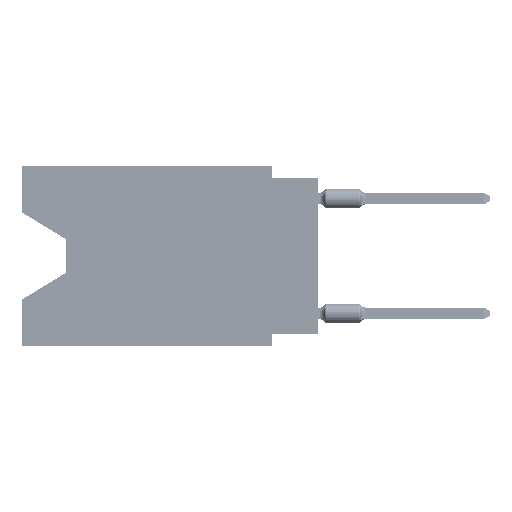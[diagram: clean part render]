
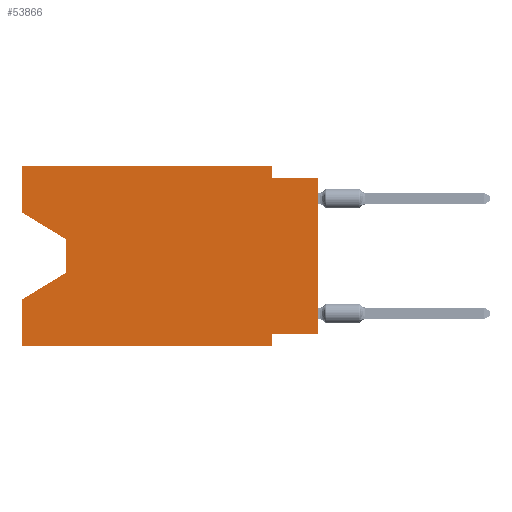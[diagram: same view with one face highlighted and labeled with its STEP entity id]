
A CAD part, left-side view. The second image highlights one B-rep face of the part: STEP entity #53866.
In plain terms, the highlighted planar face has unit normal (-1, 0, 0).
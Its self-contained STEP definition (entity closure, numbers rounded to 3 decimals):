
#454 = ORIENTED_EDGE ( 'NONE', *, *, #25153, .F. ) ;
#1083 = ORIENTED_EDGE ( 'NONE', *, *, #26147, .T. ) ;
#2957 = LINE ( 'NONE', #27052, #9145 ) ;
#4261 = LINE ( 'NONE', #43544, #16232 ) ;
#5022 = LINE ( 'NONE', #71385, #45654 ) ;
#5476 = CARTESIAN_POINT ( 'NONE',  ( 0., 16.383, 0. ) ) ;
#5584 = ORIENTED_EDGE ( 'NONE', *, *, #6152, .T. ) ;
#5935 = CARTESIAN_POINT ( 'NONE',  ( 0., 2.54, 0. ) ) ;
#5943 = DIRECTION ( 'NONE',  ( 0., 0., -1. ) ) ;
#5999 = DIRECTION ( 'NONE',  ( 0., 0., 1. ) ) ;
#6152 = EDGE_CURVE ( 'NONE', #68280, #65793, #2957, .T. ) ;
#6494 = VECTOR ( 'NONE', #56442, 1000. ) ;
#6787 = CARTESIAN_POINT ( 'NONE',  ( 0., 0., -9.271 ) ) ;
#8348 = CARTESIAN_POINT ( 'NONE',  ( 0., 2.54, -9.271 ) ) ;
#8540 = LINE ( 'NONE', #42635, #26446 ) ;
#8844 = EDGE_CURVE ( 'NONE', #23778, #34947, #56024, .T. ) ;
#9145 = VECTOR ( 'NONE', #37441, 1000. ) ;
#9618 = CARTESIAN_POINT ( 'NONE',  ( 0., 0., -9.271 ) ) ;
#10135 = CARTESIAN_POINT ( 'NONE',  ( 0., 13.97, -4.013 ) ) ;
#10814 = ORIENTED_EDGE ( 'NONE', *, *, #55298, .T. ) ;
#11912 = CARTESIAN_POINT ( 'NONE',  ( 0., 16.383, -2.546 ) ) ;
#14767 = VERTEX_POINT ( 'NONE', #33160 ) ;
#15689 = LINE ( 'NONE', #10135, #6494 ) ;
#15815 = AXIS2_PLACEMENT_3D ( 'NONE', #45076, #34333, #48904 ) ;
#16232 = VECTOR ( 'NONE', #71711, 1000. ) ;
#17795 = CARTESIAN_POINT ( 'NONE',  ( 0., 2.54, 0. ) ) ;
#19669 = ORIENTED_EDGE ( 'NONE', *, *, #37141, .F. ) ;
#21671 = CARTESIAN_POINT ( 'NONE',  ( 0., 16.383, -7.36 ) ) ;
#21964 = EDGE_CURVE ( 'NONE', #23778, #43399, #37515, .T. ) ;
#23778 = VERTEX_POINT ( 'NONE', #68617 ) ;
#23861 = ORIENTED_EDGE ( 'NONE', *, *, #24939, .T. ) ;
#24153 = VERTEX_POINT ( 'NONE', #8348 ) ;
#24939 = EDGE_CURVE ( 'NONE', #38025, #59794, #27891, .T. ) ;
#25153 = EDGE_CURVE ( 'NONE', #14767, #59794, #8540, .T. ) ;
#25950 = ORIENTED_EDGE ( 'NONE', *, *, #27632, .F. ) ;
#25965 = DIRECTION ( 'NONE',  ( 0., -1., 0. ) ) ;
#26147 = EDGE_CURVE ( 'NONE', #65669, #41123, #28624, .T. ) ;
#26446 = VECTOR ( 'NONE', #25965, 1000. ) ;
#27052 = CARTESIAN_POINT ( 'NONE',  ( 0., 16.383, -9.906 ) ) ;
#27632 = EDGE_CURVE ( 'NONE', #24153, #65793, #5022, .T. ) ;
#27891 = LINE ( 'NONE', #56785, #66697 ) ;
#28046 = VECTOR ( 'NONE', #66997, 1000. ) ;
#28202 = LINE ( 'NONE', #17795, #32927 ) ;
#28581 = VECTOR ( 'NONE', #45275, 1000. ) ;
#28624 = LINE ( 'NONE', #46400, #64419 ) ;
#30630 = VERTEX_POINT ( 'NONE', #5935 ) ;
#31551 = CARTESIAN_POINT ( 'NONE',  ( 0., 13.97, -5.893 ) ) ;
#31943 = CARTESIAN_POINT ( 'NONE',  ( 0., 16.383, 0. ) ) ;
#32927 = VECTOR ( 'NONE', #5943, 1000. ) ;
#33160 = CARTESIAN_POINT ( 'NONE',  ( 0., 2.54, -0.635 ) ) ;
#34333 = DIRECTION ( 'NONE',  ( 1., 0., 0. ) ) ;
#34562 = DIRECTION ( 'NONE',  ( 0., 0.855, -0.519 ) ) ;
#34947 = VERTEX_POINT ( 'NONE', #72459 ) ;
#35781 = EDGE_CURVE ( 'NONE', #68280, #41123, #72925, .T. ) ;
#37141 = EDGE_CURVE ( 'NONE', #30630, #14767, #28202, .T. ) ;
#37441 = DIRECTION ( 'NONE',  ( 0., -1., 0. ) ) ;
#37515 = LINE ( 'NONE', #31943, #56135 ) ;
#38025 = VERTEX_POINT ( 'NONE', #6787 ) ;
#39980 = CARTESIAN_POINT ( 'NONE',  ( 0., 16.383, -9.906 ) ) ;
#41123 = VERTEX_POINT ( 'NONE', #21671 ) ;
#42227 = CARTESIAN_POINT ( 'NONE',  ( 0., 0., -0.635 ) ) ;
#42635 = CARTESIAN_POINT ( 'NONE',  ( 0., 0., -0.635 ) ) ;
#43399 = VERTEX_POINT ( 'NONE', #53339 ) ;
#43544 = CARTESIAN_POINT ( 'NONE',  ( 0., 16.383, 0. ) ) ;
#44670 = ORIENTED_EDGE ( 'NONE', *, *, #69294, .F. ) ;
#45076 = CARTESIAN_POINT ( 'NONE',  ( 0., 16.383, 0. ) ) ;
#45275 = DIRECTION ( 'NONE',  ( 0., -0.855, -0.519 ) ) ;
#45654 = VECTOR ( 'NONE', #49516, 1000. ) ;
#46400 = CARTESIAN_POINT ( 'NONE',  ( 0., 13.97, -5.893 ) ) ;
#46787 = ORIENTED_EDGE ( 'NONE', *, *, #21964, .F. ) ;
#48904 = DIRECTION ( 'NONE',  ( 0., 0., -1. ) ) ;
#49516 = DIRECTION ( 'NONE',  ( 0., 0., -1. ) ) ;
#50369 = LINE ( 'NONE', #9618, #66965 ) ;
#53339 = CARTESIAN_POINT ( 'NONE',  ( 0., 16.383, 0. ) ) ;
#53866 = ADVANCED_FACE ( 'NONE', ( #62498 ), #71891, .F. ) ;
#55298 = EDGE_CURVE ( 'NONE', #34947, #65669, #15689, .T. ) ;
#56024 = LINE ( 'NONE', #11912, #28581 ) ;
#56135 = VECTOR ( 'NONE', #67124, 1000. ) ;
#56159 = ORIENTED_EDGE ( 'NONE', *, *, #35781, .F. ) ;
#56442 = DIRECTION ( 'NONE',  ( 0., 0., -1. ) ) ;
#56785 = CARTESIAN_POINT ( 'NONE',  ( 0., 0., 0. ) ) ;
#56894 = ORIENTED_EDGE ( 'NONE', *, *, #8844, .T. ) ;
#58615 = ORIENTED_EDGE ( 'NONE', *, *, #70048, .F. ) ;
#59794 = VERTEX_POINT ( 'NONE', #42227 ) ;
#62498 = FACE_OUTER_BOUND ( 'NONE', #66726, .T. ) ;
#62645 = CARTESIAN_POINT ( 'NONE',  ( 0., 2.54, -9.906 ) ) ;
#64419 = VECTOR ( 'NONE', #34562, 1000. ) ;
#65669 = VERTEX_POINT ( 'NONE', #31551 ) ;
#65793 = VERTEX_POINT ( 'NONE', #62645 ) ;
#66697 = VECTOR ( 'NONE', #5999, 1000. ) ;
#66726 = EDGE_LOOP ( 'NONE', ( #56894, #10814, #1083, #56159, #5584, #25950, #44670, #23861, #454, #19669, #58615, #46787 ) ) ;
#66965 = VECTOR ( 'NONE', #67396, 1000. ) ;
#66997 = DIRECTION ( 'NONE',  ( 0., 0., 1. ) ) ;
#67124 = DIRECTION ( 'NONE',  ( 0., 0., 1. ) ) ;
#67396 = DIRECTION ( 'NONE',  ( 0., 1., 0. ) ) ;
#68280 = VERTEX_POINT ( 'NONE', #39980 ) ;
#68617 = CARTESIAN_POINT ( 'NONE',  ( 0., 16.383, -2.546 ) ) ;
#69294 = EDGE_CURVE ( 'NONE', #38025, #24153, #50369, .T. ) ;
#70048 = EDGE_CURVE ( 'NONE', #43399, #30630, #4261, .T. ) ;
#71385 = CARTESIAN_POINT ( 'NONE',  ( 0., 2.54, -9.906 ) ) ;
#71711 = DIRECTION ( 'NONE',  ( 0., -1., 0. ) ) ;
#71891 = PLANE ( 'NONE',  #15815 ) ;
#72459 = CARTESIAN_POINT ( 'NONE',  ( 0., 13.97, -4.013 ) ) ;
#72925 = LINE ( 'NONE', #5476, #28046 ) ;
